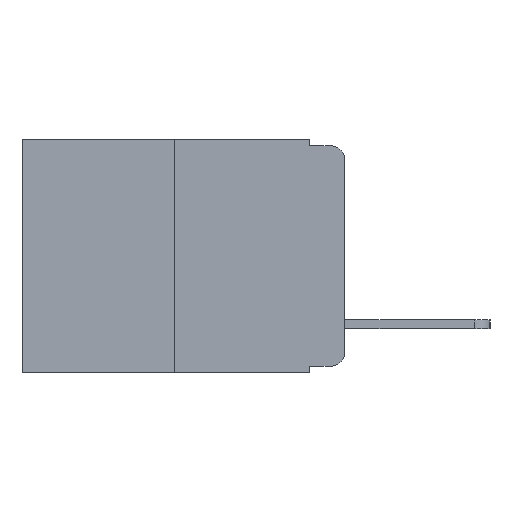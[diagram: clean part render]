
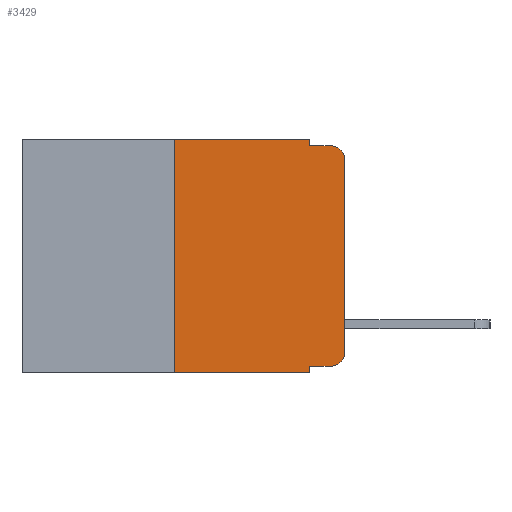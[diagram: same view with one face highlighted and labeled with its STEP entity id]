
A CAD part, left-side view. The second image highlights one B-rep face of the part: STEP entity #3429.
In plain terms, the highlighted planar face has unit normal (-1, 0, 0).
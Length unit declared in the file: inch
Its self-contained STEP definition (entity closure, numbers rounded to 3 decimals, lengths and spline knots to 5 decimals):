
#142 = EDGE_CURVE ( 'NONE', #425, #7749, #11176, .T. ) ;
#185 = DIRECTION ( 'NONE',  ( 0., 0., 1. ) ) ;
#226 = VERTEX_POINT ( 'NONE', #3223 ) ;
#311 = ORIENTED_EDGE ( 'NONE', *, *, #9561, .F. ) ;
#343 = EDGE_CURVE ( 'NONE', #226, #10621, #1441, .T. ) ;
#425 = VERTEX_POINT ( 'NONE', #10620 ) ;
#449 = EDGE_CURVE ( 'NONE', #10621, #9713, #2708, .T. ) ;
#528 = PLANE ( 'NONE',  #1523 ) ;
#532 = ORIENTED_EDGE ( 'NONE', *, *, #449, .T. ) ;
#577 = CARTESIAN_POINT ( 'NONE',  ( 0., 0.051, 0. ) ) ;
#722 = EDGE_CURVE ( 'NONE', #425, #11571, #11584, .T. ) ;
#803 = EDGE_LOOP ( 'NONE', ( #5506, #6100, #6921, #8616, #311, #3160, #4109, #7492, #6757, #532 ) ) ;
#839 = VERTEX_POINT ( 'NONE', #6800 ) ;
#1013 = CARTESIAN_POINT ( 'NONE',  ( 0., 0.473, 0. ) ) ;
#1153 = CARTESIAN_POINT ( 'NONE',  ( 0., 0.02, -0.03 ) ) ;
#1210 = AXIS2_PLACEMENT_3D ( 'NONE', #1153, #8158, #2354 ) ;
#1408 = EDGE_CURVE ( 'NONE', #226, #11571, #8361, .T. ) ;
#1441 = LINE ( 'NONE', #5633, #7143 ) ;
#1523 = AXIS2_PLACEMENT_3D ( 'NONE', #1013, #4529, #5651 ) ;
#1530 = CARTESIAN_POINT ( 'NONE',  ( 0., 0., 0. ) ) ;
#1604 = EDGE_CURVE ( 'NONE', #5047, #4718, #10572, .T. ) ;
#1627 = DIRECTION ( 'NONE',  ( 0., -1., 0. ) ) ;
#2288 = EDGE_CURVE ( 'NONE', #4718, #839, #9821, .T. ) ;
#2354 = DIRECTION ( 'NONE',  ( 0., 0., -1. ) ) ;
#2708 = CIRCLE ( 'NONE', #8155, 0.02 ) ;
#3160 = ORIENTED_EDGE ( 'NONE', *, *, #142, .F. ) ;
#3223 = CARTESIAN_POINT ( 'NONE',  ( 0., 0.051, -0.333 ) ) ;
#3429 = ADVANCED_FACE ( 'NONE', ( #5237 ), #528, .F. ) ;
#3643 = EDGE_CURVE ( 'NONE', #11298, #839, #11962, .T. ) ;
#3938 = VECTOR ( 'NONE', #8137, 39.37008 ) ;
#3945 = EDGE_CURVE ( 'NONE', #9713, #11298, #10316, .T. ) ;
#4109 = ORIENTED_EDGE ( 'NONE', *, *, #722, .T. ) ;
#4529 = DIRECTION ( 'NONE',  ( 1., 0., 0. ) ) ;
#4718 = VERTEX_POINT ( 'NONE', #9317 ) ;
#4970 = CARTESIAN_POINT ( 'NONE',  ( 0., 0.051, -0.01 ) ) ;
#4994 = VECTOR ( 'NONE', #1627, 39.37008 ) ;
#5047 = VERTEX_POINT ( 'NONE', #577 ) ;
#5083 = DIRECTION ( 'NONE',  ( 0., -1., 0. ) ) ;
#5237 = FACE_OUTER_BOUND ( 'NONE', #803, .T. ) ;
#5378 = DIRECTION ( 'NONE',  ( 0., -1., 0. ) ) ;
#5506 = ORIENTED_EDGE ( 'NONE', *, *, #3945, .T. ) ;
#5633 = CARTESIAN_POINT ( 'NONE',  ( 0., 0.051, -0.333 ) ) ;
#5651 = DIRECTION ( 'NONE',  ( 0., 0., -1. ) ) ;
#6100 = ORIENTED_EDGE ( 'NONE', *, *, #3643, .T. ) ;
#6337 = CARTESIAN_POINT ( 'NONE',  ( 0., 0.473, 0. ) ) ;
#6757 = ORIENTED_EDGE ( 'NONE', *, *, #343, .T. ) ;
#6800 = CARTESIAN_POINT ( 'NONE',  ( 0., 0.02, -0.01 ) ) ;
#6921 = ORIENTED_EDGE ( 'NONE', *, *, #2288, .F. ) ;
#7143 = VECTOR ( 'NONE', #5083, 39.37008 ) ;
#7360 = CARTESIAN_POINT ( 'NONE',  ( 0., 0.02, -0.333 ) ) ;
#7492 = ORIENTED_EDGE ( 'NONE', *, *, #1408, .F. ) ;
#7703 = CARTESIAN_POINT ( 'NONE',  ( 0., 0.02, -0.313 ) ) ;
#7749 = VERTEX_POINT ( 'NONE', #12549 ) ;
#7754 = CARTESIAN_POINT ( 'NONE',  ( 0., 0., -0.313 ) ) ;
#8137 = DIRECTION ( 'NONE',  ( 0., 0., 1. ) ) ;
#8155 = AXIS2_PLACEMENT_3D ( 'NONE', #7703, #10789, #9278 ) ;
#8158 = DIRECTION ( 'NONE',  ( -1., 0., 0. ) ) ;
#8361 = LINE ( 'NONE', #11358, #10446 ) ;
#8441 = CARTESIAN_POINT ( 'NONE',  ( 0., 0.25, 0. ) ) ;
#8616 = ORIENTED_EDGE ( 'NONE', *, *, #1604, .F. ) ;
#8967 = DIRECTION ( 'NONE',  ( 0., -1., 0. ) ) ;
#9245 = VECTOR ( 'NONE', #8967, 39.37008 ) ;
#9278 = DIRECTION ( 'NONE',  ( 0., 0., -1. ) ) ;
#9317 = CARTESIAN_POINT ( 'NONE',  ( 0., 0.051, -0.01 ) ) ;
#9417 = DIRECTION ( 'NONE',  ( 0., 0., -1. ) ) ;
#9428 = CARTESIAN_POINT ( 'NONE',  ( 0., 0.051, -0.343 ) ) ;
#9430 = CARTESIAN_POINT ( 'NONE',  ( 0., 0.051, 0. ) ) ;
#9561 = EDGE_CURVE ( 'NONE', #7749, #5047, #9593, .T. ) ;
#9593 = LINE ( 'NONE', #6337, #11380 ) ;
#9713 = VERTEX_POINT ( 'NONE', #7754 ) ;
#9781 = CARTESIAN_POINT ( 'NONE',  ( 0., 0.473, -0.343 ) ) ;
#9821 = LINE ( 'NONE', #4970, #4994 ) ;
#9842 = VECTOR ( 'NONE', #9417, 39.37008 ) ;
#10316 = LINE ( 'NONE', #1530, #12358 ) ;
#10446 = VECTOR ( 'NONE', #11272, 39.37008 ) ;
#10572 = LINE ( 'NONE', #9430, #9842 ) ;
#10620 = CARTESIAN_POINT ( 'NONE',  ( 0., 0.25, -0.343 ) ) ;
#10621 = VERTEX_POINT ( 'NONE', #7360 ) ;
#10789 = DIRECTION ( 'NONE',  ( -1., 0., 0. ) ) ;
#11176 = LINE ( 'NONE', #8441, #3938 ) ;
#11272 = DIRECTION ( 'NONE',  ( 0., 0., -1. ) ) ;
#11298 = VERTEX_POINT ( 'NONE', #12507 ) ;
#11358 = CARTESIAN_POINT ( 'NONE',  ( 0., 0.051, 0. ) ) ;
#11380 = VECTOR ( 'NONE', #5378, 39.37008 ) ;
#11571 = VERTEX_POINT ( 'NONE', #9428 ) ;
#11584 = LINE ( 'NONE', #9781, #9245 ) ;
#11962 = CIRCLE ( 'NONE', #1210, 0.02 ) ;
#12358 = VECTOR ( 'NONE', #185, 39.37008 ) ;
#12507 = CARTESIAN_POINT ( 'NONE',  ( 0., 0., -0.03 ) ) ;
#12549 = CARTESIAN_POINT ( 'NONE',  ( 0., 0.25, 0. ) ) ;
